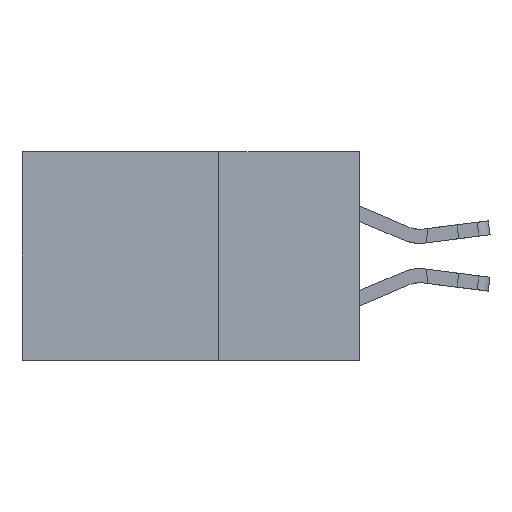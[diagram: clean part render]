
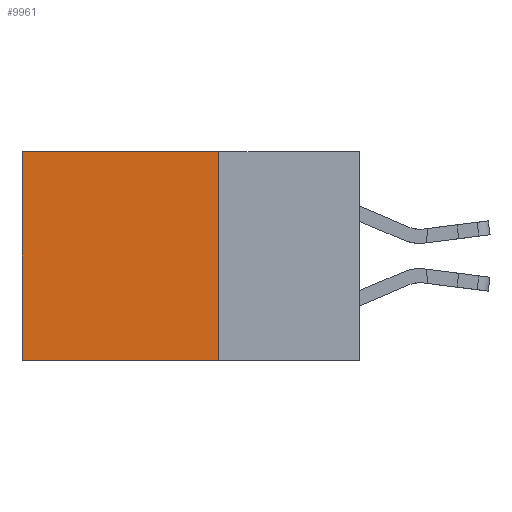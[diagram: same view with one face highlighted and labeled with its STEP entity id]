
A CAD part, left-side view. The second image highlights one B-rep face of the part: STEP entity #9961.
In plain terms, the highlighted planar face has unit normal (-1, 0, 0).
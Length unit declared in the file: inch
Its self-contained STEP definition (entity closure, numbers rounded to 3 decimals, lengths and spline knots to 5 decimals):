
#79 = CARTESIAN_POINT ( 'NONE',  ( 0.2875, 0.25, 0. ) ) ;
#720 = VECTOR ( 'NONE', #10055, 39.37008 ) ;
#1894 = VECTOR ( 'NONE', #3346, 39.37008 ) ;
#1968 = EDGE_LOOP ( 'NONE', ( #13521, #24953, #16055, #21061 ) ) ;
#2186 = CARTESIAN_POINT ( 'NONE',  ( 0.2875, 0.25, 0. ) ) ;
#2473 = DIRECTION ( 'NONE',  ( 1., 0., 0. ) ) ;
#2651 = DIRECTION ( 'NONE',  ( 0., 0., -1. ) ) ;
#2766 = VERTEX_POINT ( 'NONE', #79 ) ;
#3346 = DIRECTION ( 'NONE',  ( 0., 0., -1. ) ) ;
#3916 = EDGE_CURVE ( 'NONE', #12627, #11269, #5754, .T. ) ;
#4970 = EDGE_CURVE ( 'NONE', #2766, #12627, #13379, .T. ) ;
#5049 = DIRECTION ( 'NONE',  ( 0., 1., 0. ) ) ;
#5754 = LINE ( 'NONE', #10243, #720 ) ;
#6956 = LINE ( 'NONE', #16132, #1894 ) ;
#9049 = CARTESIAN_POINT ( 'NONE',  ( 0.2875, 0.25, 0. ) ) ;
#9431 = VECTOR ( 'NONE', #5049, 39.37008 ) ;
#9961 = ADVANCED_FACE ( 'NONE', ( #15158 ), #11182, .F. ) ;
#10055 = DIRECTION ( 'NONE',  ( 0., 0., -1. ) ) ;
#10243 = CARTESIAN_POINT ( 'NONE',  ( 0.2875, 0.6, 0. ) ) ;
#11131 = CARTESIAN_POINT ( 'NONE',  ( 0.2875, 0.25, -0.37 ) ) ;
#11182 = PLANE ( 'NONE',  #15504 ) ;
#11269 = VERTEX_POINT ( 'NONE', #24868 ) ;
#12627 = VERTEX_POINT ( 'NONE', #13634 ) ;
#13379 = LINE ( 'NONE', #2186, #21059 ) ;
#13521 = ORIENTED_EDGE ( 'NONE', *, *, #3916, .T. ) ;
#13634 = CARTESIAN_POINT ( 'NONE',  ( 0.2875, 0.6, 0. ) ) ;
#15014 = DIRECTION ( 'NONE',  ( 0., 1., 0. ) ) ;
#15158 = FACE_OUTER_BOUND ( 'NONE', #1968, .T. ) ;
#15504 = AXIS2_PLACEMENT_3D ( 'NONE', #9049, #2473, #2651 ) ;
#16055 = ORIENTED_EDGE ( 'NONE', *, *, #21404, .F. ) ;
#16132 = CARTESIAN_POINT ( 'NONE',  ( 0.2875, 0.25, 0. ) ) ;
#17006 = CARTESIAN_POINT ( 'NONE',  ( 0.2875, 0.25, -0.37 ) ) ;
#20986 = VERTEX_POINT ( 'NONE', #17006 ) ;
#21059 = VECTOR ( 'NONE', #15014, 39.37008 ) ;
#21061 = ORIENTED_EDGE ( 'NONE', *, *, #4970, .T. ) ;
#21404 = EDGE_CURVE ( 'NONE', #2766, #20986, #6956, .T. ) ;
#22075 = LINE ( 'NONE', #11131, #9431 ) ;
#24868 = CARTESIAN_POINT ( 'NONE',  ( 0.2875, 0.6, -0.37 ) ) ;
#24953 = ORIENTED_EDGE ( 'NONE', *, *, #25051, .F. ) ;
#25051 = EDGE_CURVE ( 'NONE', #20986, #11269, #22075, .T. ) ;
